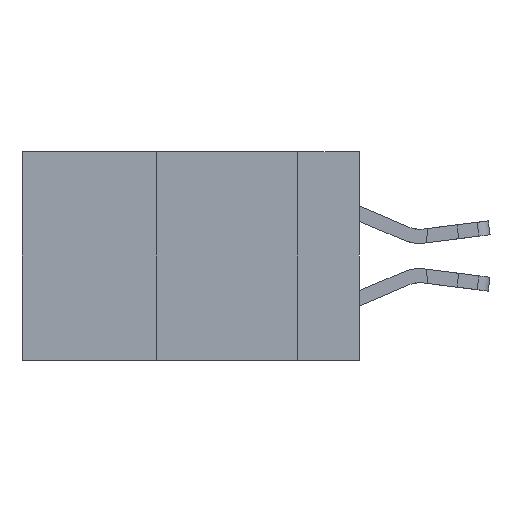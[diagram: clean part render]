
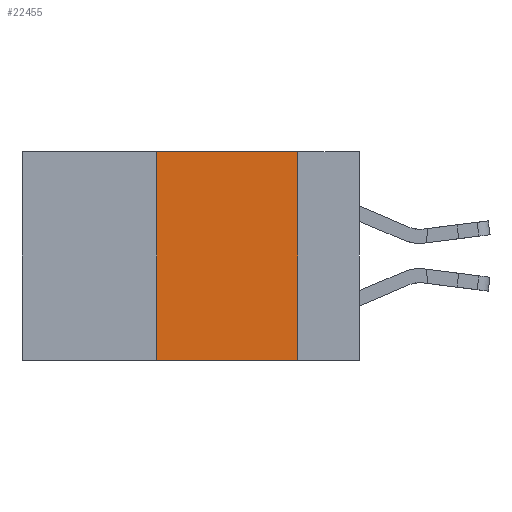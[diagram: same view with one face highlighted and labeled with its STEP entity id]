
A CAD part, left-side view. The second image highlights one B-rep face of the part: STEP entity #22455.
In plain terms, the highlighted planar face has unit normal (-1, 0, 0).
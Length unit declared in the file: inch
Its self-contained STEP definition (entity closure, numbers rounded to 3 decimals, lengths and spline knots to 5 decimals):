
#84 = VECTOR ( 'NONE', #2032, 39.37008 ) ;
#754 = DIRECTION ( 'NONE',  ( 0., 0., -1. ) ) ;
#912 = CARTESIAN_POINT ( 'NONE',  ( 0., 0.11, 0. ) ) ;
#1177 = VECTOR ( 'NONE', #8246, 39.37008 ) ;
#2032 = DIRECTION ( 'NONE',  ( 0., -1., 0. ) ) ;
#2088 = CARTESIAN_POINT ( 'NONE',  ( 0., 0.11, 0. ) ) ;
#3422 = EDGE_CURVE ( 'NONE', #8472, #17839, #20202, .T. ) ;
#3906 = EDGE_LOOP ( 'NONE', ( #17868, #18137, #15286, #4724 ) ) ;
#4617 = DIRECTION ( 'NONE',  ( 0., 0., 1. ) ) ;
#4724 = ORIENTED_EDGE ( 'NONE', *, *, #14069, .T. ) ;
#5995 = CARTESIAN_POINT ( 'NONE',  ( 0., 0.6, -0.37 ) ) ;
#6507 = CARTESIAN_POINT ( 'NONE',  ( 0., 0.6, 0. ) ) ;
#7052 = CARTESIAN_POINT ( 'NONE',  ( 0., 0.36, -0.37 ) ) ;
#8246 = DIRECTION ( 'NONE',  ( 0., -1., 0. ) ) ;
#8472 = VERTEX_POINT ( 'NONE', #7052 ) ;
#8582 = CARTESIAN_POINT ( 'NONE',  ( 0., 0.6, 0. ) ) ;
#9633 = LINE ( 'NONE', #8582, #1177 ) ;
#10533 = CARTESIAN_POINT ( 'NONE',  ( 0., 0.36, 0. ) ) ;
#10591 = EDGE_CURVE ( 'NONE', #22997, #18163, #10606, .T. ) ;
#10606 = LINE ( 'NONE', #912, #15690 ) ;
#11693 = EDGE_CURVE ( 'NONE', #17839, #22997, #9633, .T. ) ;
#12601 = DIRECTION ( 'NONE',  ( 0., 0., -1. ) ) ;
#14069 = EDGE_CURVE ( 'NONE', #8472, #18163, #15443, .T. ) ;
#14219 = DIRECTION ( 'NONE',  ( 1., 0., 0. ) ) ;
#14414 = VECTOR ( 'NONE', #4617, 39.37008 ) ;
#15286 = ORIENTED_EDGE ( 'NONE', *, *, #3422, .F. ) ;
#15443 = LINE ( 'NONE', #5995, #84 ) ;
#15690 = VECTOR ( 'NONE', #12601, 39.37008 ) ;
#15981 = PLANE ( 'NONE',  #17892 ) ;
#17839 = VERTEX_POINT ( 'NONE', #10533 ) ;
#17868 = ORIENTED_EDGE ( 'NONE', *, *, #10591, .F. ) ;
#17892 = AXIS2_PLACEMENT_3D ( 'NONE', #6507, #14219, #754 ) ;
#18137 = ORIENTED_EDGE ( 'NONE', *, *, #11693, .F. ) ;
#18163 = VERTEX_POINT ( 'NONE', #19209 ) ;
#19209 = CARTESIAN_POINT ( 'NONE',  ( 0., 0.11, -0.37 ) ) ;
#20202 = LINE ( 'NONE', #23707, #14414 ) ;
#20330 = FACE_OUTER_BOUND ( 'NONE', #3906, .T. ) ;
#22455 = ADVANCED_FACE ( 'NONE', ( #20330 ), #15981, .F. ) ;
#22997 = VERTEX_POINT ( 'NONE', #2088 ) ;
#23707 = CARTESIAN_POINT ( 'NONE',  ( 0., 0.36, 0. ) ) ;
